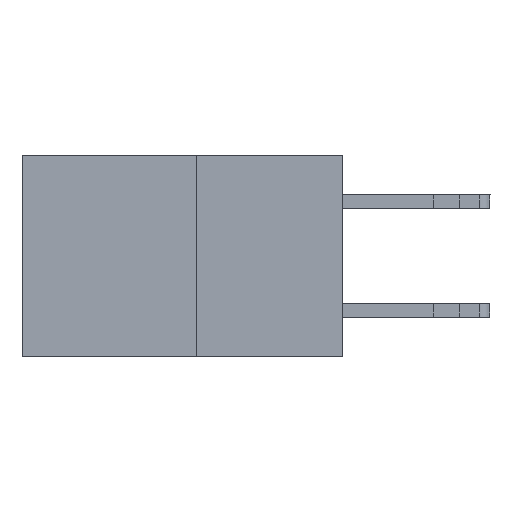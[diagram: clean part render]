
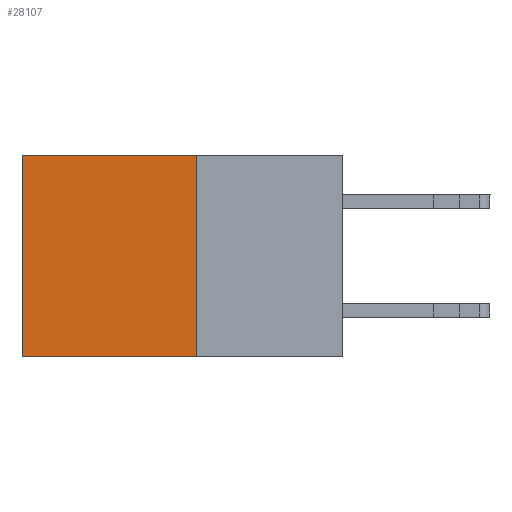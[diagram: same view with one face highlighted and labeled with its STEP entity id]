
A CAD part, left-side view. The second image highlights one B-rep face of the part: STEP entity #28107.
In plain terms, the highlighted planar face has unit normal (-1, 0, 0).
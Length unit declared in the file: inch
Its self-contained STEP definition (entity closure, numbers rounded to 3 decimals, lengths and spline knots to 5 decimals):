
#231 = DIRECTION ( 'NONE',  ( 0., 1., 0. ) ) ;
#920 = DIRECTION ( 'NONE',  ( 0., 0., -1. ) ) ;
#1220 = PLANE ( 'NONE',  #21256 ) ;
#3155 = LINE ( 'NONE', #3601, #18785 ) ;
#3601 = CARTESIAN_POINT ( 'NONE',  ( 0.277, 0.27, -0.37 ) ) ;
#3932 = DIRECTION ( 'NONE',  ( 0., 0., -1. ) ) ;
#4079 = ORIENTED_EDGE ( 'NONE', *, *, #11291, .T. ) ;
#4975 = VERTEX_POINT ( 'NONE', #22985 ) ;
#5515 = LINE ( 'NONE', #20396, #27720 ) ;
#7053 = EDGE_CURVE ( 'NONE', #21244, #4975, #11069, .T. ) ;
#10497 = EDGE_LOOP ( 'NONE', ( #4079, #19809, #13039, #23326 ) ) ;
#11069 = LINE ( 'NONE', #17724, #16536 ) ;
#11291 = EDGE_CURVE ( 'NONE', #4975, #25312, #5515, .T. ) ;
#11345 = CARTESIAN_POINT ( 'NONE',  ( 0.277, 0.27, 0. ) ) ;
#11870 = DIRECTION ( 'NONE',  ( 0., 0., -1. ) ) ;
#13039 = ORIENTED_EDGE ( 'NONE', *, *, #20425, .F. ) ;
#13514 = DIRECTION ( 'NONE',  ( 1., 0., 0. ) ) ;
#15052 = LINE ( 'NONE', #19381, #24733 ) ;
#16536 = VECTOR ( 'NONE', #231, 39.37008 ) ;
#17724 = CARTESIAN_POINT ( 'NONE',  ( 0.277, 0.27, 0. ) ) ;
#18785 = VECTOR ( 'NONE', #18915, 39.37008 ) ;
#18915 = DIRECTION ( 'NONE',  ( 0., 1., 0. ) ) ;
#19381 = CARTESIAN_POINT ( 'NONE',  ( 0.277, 0.27, -0.37 ) ) ;
#19461 = CARTESIAN_POINT ( 'NONE',  ( 0.277, 0.27, -0.37 ) ) ;
#19809 = ORIENTED_EDGE ( 'NONE', *, *, #23599, .F. ) ;
#20396 = CARTESIAN_POINT ( 'NONE',  ( 0.277, 0.59, -0.37 ) ) ;
#20425 = EDGE_CURVE ( 'NONE', #21244, #25000, #15052, .T. ) ;
#21244 = VERTEX_POINT ( 'NONE', #11345 ) ;
#21256 = AXIS2_PLACEMENT_3D ( 'NONE', #22903, #13514, #920 ) ;
#22903 = CARTESIAN_POINT ( 'NONE',  ( 0.277, 0.27, -0.37 ) ) ;
#22985 = CARTESIAN_POINT ( 'NONE',  ( 0.277, 0.59, 0. ) ) ;
#23326 = ORIENTED_EDGE ( 'NONE', *, *, #7053, .T. ) ;
#23599 = EDGE_CURVE ( 'NONE', #25000, #25312, #3155, .T. ) ;
#24733 = VECTOR ( 'NONE', #3932, 39.37008 ) ;
#25000 = VERTEX_POINT ( 'NONE', #19461 ) ;
#25213 = FACE_OUTER_BOUND ( 'NONE', #10497, .T. ) ;
#25312 = VERTEX_POINT ( 'NONE', #27255 ) ;
#27255 = CARTESIAN_POINT ( 'NONE',  ( 0.277, 0.59, -0.37 ) ) ;
#27720 = VECTOR ( 'NONE', #11870, 39.37008 ) ;
#28107 = ADVANCED_FACE ( 'NONE', ( #25213 ), #1220, .F. ) ;
